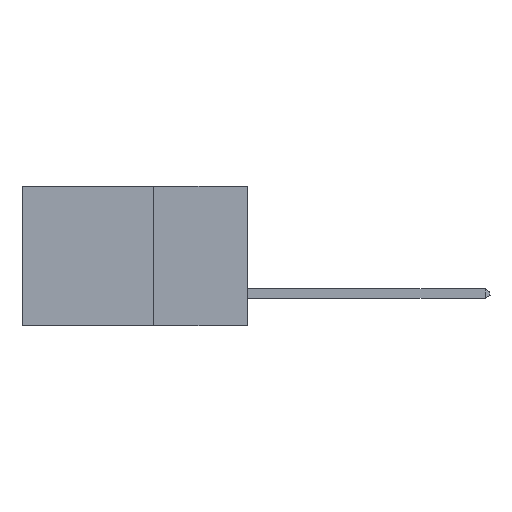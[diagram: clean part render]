
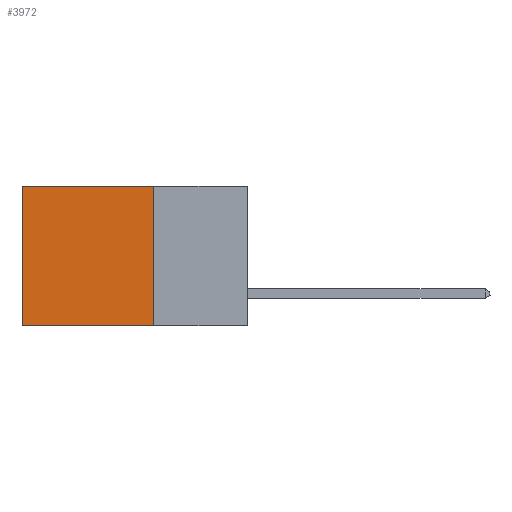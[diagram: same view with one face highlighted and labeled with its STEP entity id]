
A CAD part, left-side view. The second image highlights one B-rep face of the part: STEP entity #3972.
In plain terms, the highlighted planar face has unit normal (-1, 0, 0).
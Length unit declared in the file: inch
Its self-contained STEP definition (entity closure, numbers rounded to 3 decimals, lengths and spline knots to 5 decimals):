
#406 = EDGE_CURVE ( 'NONE', #16290, #6220, #10472, .T. ) ;
#784 = LINE ( 'NONE', #10610, #22118 ) ;
#1378 = LINE ( 'NONE', #5061, #7125 ) ;
#1970 = DIRECTION ( 'NONE',  ( 0., 1., 0. ) ) ;
#2754 = CARTESIAN_POINT ( 'NONE',  ( 0.298, 0.25, -0.37 ) ) ;
#3287 = FACE_OUTER_BOUND ( 'NONE', #11027, .T. ) ;
#3690 = EDGE_CURVE ( 'NONE', #4801, #19257, #784, .T. ) ;
#3972 = ADVANCED_FACE ( 'NONE', ( #3287 ), #11575, .F. ) ;
#4000 = DIRECTION ( 'NONE',  ( 0., 1., 0. ) ) ;
#4332 = ORIENTED_EDGE ( 'NONE', *, *, #21942, .T. ) ;
#4801 = VERTEX_POINT ( 'NONE', #2754 ) ;
#5061 = CARTESIAN_POINT ( 'NONE',  ( 0.298, 0.6, 0. ) ) ;
#5611 = DIRECTION ( 'NONE',  ( 0., 0., -1. ) ) ;
#6220 = VERTEX_POINT ( 'NONE', #12202 ) ;
#6614 = CARTESIAN_POINT ( 'NONE',  ( 0.298, 0.25, 0. ) ) ;
#7125 = VECTOR ( 'NONE', #17017, 39.37008 ) ;
#8084 = DIRECTION ( 'NONE',  ( 1., 0., 0. ) ) ;
#9601 = LINE ( 'NONE', #12405, #21700 ) ;
#9666 = CARTESIAN_POINT ( 'NONE',  ( 0.298, 0.25, 0. ) ) ;
#10472 = LINE ( 'NONE', #12428, #15703 ) ;
#10610 = CARTESIAN_POINT ( 'NONE',  ( 0.298, 0.25, -0.37 ) ) ;
#10986 = ORIENTED_EDGE ( 'NONE', *, *, #20208, .F. ) ;
#11027 = EDGE_LOOP ( 'NONE', ( #4332, #18862, #10986, #12467 ) ) ;
#11346 = DIRECTION ( 'NONE',  ( 0., 0., -1. ) ) ;
#11575 = PLANE ( 'NONE',  #19021 ) ;
#12202 = CARTESIAN_POINT ( 'NONE',  ( 0.298, 0.6, 0. ) ) ;
#12405 = CARTESIAN_POINT ( 'NONE',  ( 0.298, 0.25, 0. ) ) ;
#12428 = CARTESIAN_POINT ( 'NONE',  ( 0.298, 0.25, 0. ) ) ;
#12467 = ORIENTED_EDGE ( 'NONE', *, *, #406, .T. ) ;
#15703 = VECTOR ( 'NONE', #4000, 39.37008 ) ;
#16066 = CARTESIAN_POINT ( 'NONE',  ( 0.298, 0.6, -0.37 ) ) ;
#16290 = VERTEX_POINT ( 'NONE', #6614 ) ;
#17017 = DIRECTION ( 'NONE',  ( 0., 0., -1. ) ) ;
#18862 = ORIENTED_EDGE ( 'NONE', *, *, #3690, .F. ) ;
#19021 = AXIS2_PLACEMENT_3D ( 'NONE', #9666, #8084, #11346 ) ;
#19257 = VERTEX_POINT ( 'NONE', #16066 ) ;
#20208 = EDGE_CURVE ( 'NONE', #16290, #4801, #9601, .T. ) ;
#21700 = VECTOR ( 'NONE', #5611, 39.37008 ) ;
#21942 = EDGE_CURVE ( 'NONE', #6220, #19257, #1378, .T. ) ;
#22118 = VECTOR ( 'NONE', #1970, 39.37008 ) ;
